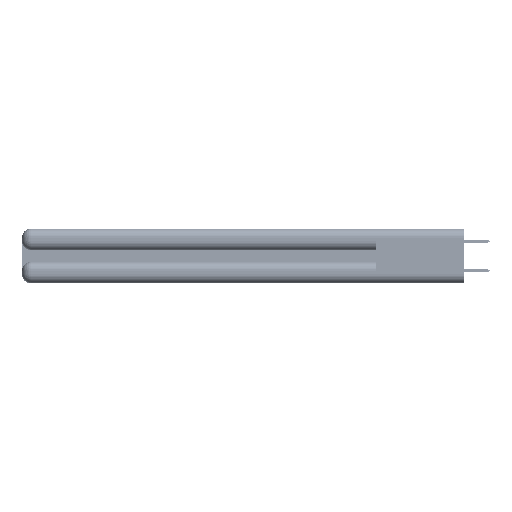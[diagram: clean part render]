
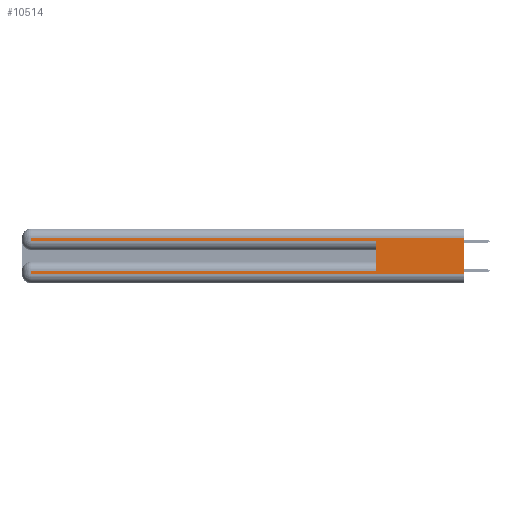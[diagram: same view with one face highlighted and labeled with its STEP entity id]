
A CAD part, left-side view. The second image highlights one B-rep face of the part: STEP entity #10514.
In plain terms, the highlighted planar face has unit normal (-1, 0, 0).
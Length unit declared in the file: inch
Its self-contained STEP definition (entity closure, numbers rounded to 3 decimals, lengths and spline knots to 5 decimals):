
#666 = EDGE_CURVE ( 'NONE', #42704, #12829, #8566, .T. ) ;
#4483 = CARTESIAN_POINT ( 'NONE',  ( 0., 2.94, 0.285 ) ) ;
#5331 = CARTESIAN_POINT ( 'NONE',  ( 0., 0., 0.285 ) ) ;
#5520 = EDGE_CURVE ( 'NONE', #34752, #42704, #43076, .T. ) ;
#7065 = LINE ( 'NONE', #30015, #39306 ) ;
#8019 = VERTEX_POINT ( 'NONE', #27881 ) ;
#8566 = LINE ( 'NONE', #5331, #18416 ) ;
#9013 = DIRECTION ( 'NONE',  ( 0., 0., -1. ) ) ;
#9388 = VECTOR ( 'NONE', #40638, 39.37008 ) ;
#10294 = VECTOR ( 'NONE', #42728, 39.37008 ) ;
#10514 = ADVANCED_FACE ( 'NONE', ( #21384 ), #32505, .F. ) ;
#11190 = CARTESIAN_POINT ( 'NONE',  ( 0., 0.6, 0.145 ) ) ;
#11780 = CARTESIAN_POINT ( 'NONE',  ( 0., 0., 0.31 ) ) ;
#12506 = EDGE_CURVE ( 'NONE', #32879, #46132, #38873, .T. ) ;
#12829 = VERTEX_POINT ( 'NONE', #31299 ) ;
#12840 = EDGE_LOOP ( 'NONE', ( #35067, #13961, #17904, #23931, #25360, #26038, #27417, #29279 ) ) ;
#12898 = DIRECTION ( 'NONE',  ( 0., 1., 0. ) ) ;
#13961 = ORIENTED_EDGE ( 'NONE', *, *, #38403, .T. ) ;
#14673 = EDGE_CURVE ( 'NONE', #31440, #32879, #43895, .T. ) ;
#17120 = CARTESIAN_POINT ( 'NONE',  ( 0., 0., 0.085 ) ) ;
#17904 = ORIENTED_EDGE ( 'NONE', *, *, #5520, .T. ) ;
#18416 = VECTOR ( 'NONE', #30509, 39.37008 ) ;
#18958 = VECTOR ( 'NONE', #28116, 39.37008 ) ;
#20218 = EDGE_CURVE ( 'NONE', #8019, #12829, #40078, .T. ) ;
#21384 = FACE_OUTER_BOUND ( 'NONE', #12840, .T. ) ;
#23771 = DIRECTION ( 'NONE',  ( 0., -1., 0. ) ) ;
#23931 = ORIENTED_EDGE ( 'NONE', *, *, #666, .T. ) ;
#24229 = CARTESIAN_POINT ( 'NONE',  ( 0., 0., 0.37 ) ) ;
#25360 = ORIENTED_EDGE ( 'NONE', *, *, #20218, .F. ) ;
#26038 = ORIENTED_EDGE ( 'NONE', *, *, #36979, .T. ) ;
#26590 = LINE ( 'NONE', #17120, #47725 ) ;
#27417 = ORIENTED_EDGE ( 'NONE', *, *, #14673, .T. ) ;
#27667 = VECTOR ( 'NONE', #23771, 39.37008 ) ;
#27881 = CARTESIAN_POINT ( 'NONE',  ( 0., 0.6, 0.085 ) ) ;
#28116 = DIRECTION ( 'NONE',  ( 0., 0., 1. ) ) ;
#28467 = DIRECTION ( 'NONE',  ( 0., 0., -1. ) ) ;
#29279 = ORIENTED_EDGE ( 'NONE', *, *, #12506, .T. ) ;
#30015 = CARTESIAN_POINT ( 'NONE',  ( 0., 0., 0.37 ) ) ;
#30509 = DIRECTION ( 'NONE',  ( 0., -1., 0. ) ) ;
#31299 = CARTESIAN_POINT ( 'NONE',  ( 0., 0.6, 0.285 ) ) ;
#31440 = VERTEX_POINT ( 'NONE', #54401 ) ;
#31794 = LINE ( 'NONE', #40464, #9388 ) ;
#32505 = PLANE ( 'NONE',  #49362 ) ;
#32879 = VERTEX_POINT ( 'NONE', #34478 ) ;
#34478 = CARTESIAN_POINT ( 'NONE',  ( 0., 2.94, 0.06 ) ) ;
#34752 = VERTEX_POINT ( 'NONE', #52738 ) ;
#35067 = ORIENTED_EDGE ( 'NONE', *, *, #50995, .F. ) ;
#36979 = EDGE_CURVE ( 'NONE', #8019, #31440, #26590, .T. ) ;
#38403 = EDGE_CURVE ( 'NONE', #48036, #34752, #31794, .T. ) ;
#38491 = CARTESIAN_POINT ( 'NONE',  ( 0., 2.94, 0.37 ) ) ;
#38873 = LINE ( 'NONE', #40362, #27667 ) ;
#39306 = VECTOR ( 'NONE', #9013, 39.37008 ) ;
#40078 = LINE ( 'NONE', #11190, #18958 ) ;
#40272 = DIRECTION ( 'NONE',  ( 0., 0., -1. ) ) ;
#40362 = CARTESIAN_POINT ( 'NONE',  ( 0., 0., 0.06 ) ) ;
#40464 = CARTESIAN_POINT ( 'NONE',  ( 0., 0., 0.31 ) ) ;
#40638 = DIRECTION ( 'NONE',  ( 0., 1., 0. ) ) ;
#42704 = VERTEX_POINT ( 'NONE', #4483 ) ;
#42728 = DIRECTION ( 'NONE',  ( 0., 0., -1. ) ) ;
#43076 = LINE ( 'NONE', #44331, #52976 ) ;
#43895 = LINE ( 'NONE', #38491, #10294 ) ;
#44331 = CARTESIAN_POINT ( 'NONE',  ( 0., 2.94, 0.37 ) ) ;
#45459 = CARTESIAN_POINT ( 'NONE',  ( 0., 0., 0.06 ) ) ;
#46132 = VERTEX_POINT ( 'NONE', #45459 ) ;
#47725 = VECTOR ( 'NONE', #12898, 39.37008 ) ;
#48036 = VERTEX_POINT ( 'NONE', #11780 ) ;
#49362 = AXIS2_PLACEMENT_3D ( 'NONE', #24229, #53672, #28467 ) ;
#50995 = EDGE_CURVE ( 'NONE', #48036, #46132, #7065, .T. ) ;
#52738 = CARTESIAN_POINT ( 'NONE',  ( 0., 2.94, 0.31 ) ) ;
#52976 = VECTOR ( 'NONE', #40272, 39.37008 ) ;
#53672 = DIRECTION ( 'NONE',  ( 1., 0., 0. ) ) ;
#54401 = CARTESIAN_POINT ( 'NONE',  ( 0., 2.94, 0.085 ) ) ;
